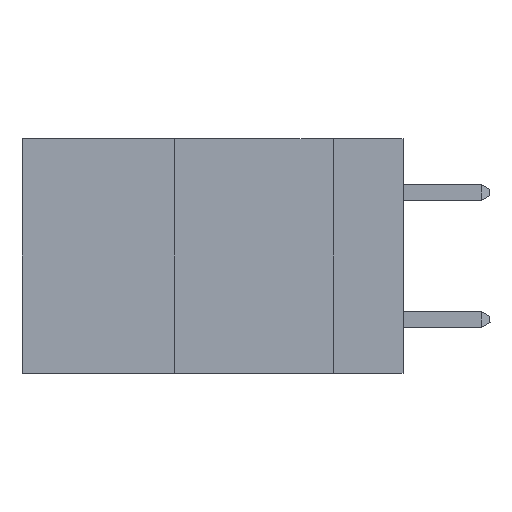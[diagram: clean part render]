
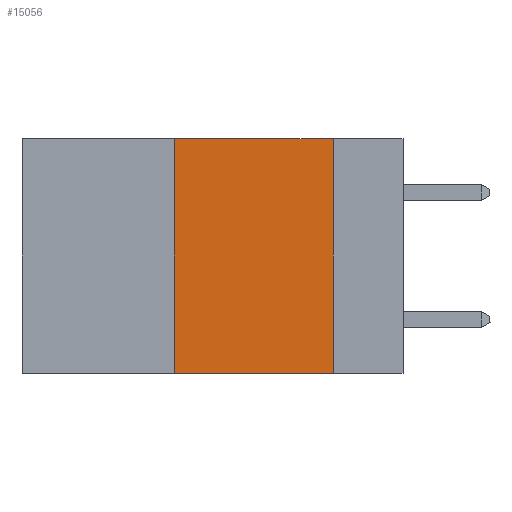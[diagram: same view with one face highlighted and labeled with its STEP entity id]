
A CAD part, left-side view. The second image highlights one B-rep face of the part: STEP entity #15056.
In plain terms, the highlighted planar face has unit normal (-1, 0, 0).
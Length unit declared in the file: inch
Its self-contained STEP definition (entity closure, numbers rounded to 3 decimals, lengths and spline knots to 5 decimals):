
#1637 = LINE ( 'NONE', #20381, #5065 ) ;
#2630 = EDGE_CURVE ( 'NONE', #11672, #5572, #18653, .T. ) ;
#3576 = CARTESIAN_POINT ( 'NONE',  ( 0., 0.36, 0. ) ) ;
#3713 = ORIENTED_EDGE ( 'NONE', *, *, #13079, .F. ) ;
#3814 = ORIENTED_EDGE ( 'NONE', *, *, #17910, .F. ) ;
#4360 = CARTESIAN_POINT ( 'NONE',  ( 0., 0.11, 0. ) ) ;
#4587 = CARTESIAN_POINT ( 'NONE',  ( 0., 0.36, -0.37 ) ) ;
#4958 = LINE ( 'NONE', #16543, #14287 ) ;
#5065 = VECTOR ( 'NONE', #20529, 39.37008 ) ;
#5572 = VERTEX_POINT ( 'NONE', #16097 ) ;
#6463 = CARTESIAN_POINT ( 'NONE',  ( 0., 0.6, -0.37 ) ) ;
#6988 = AXIS2_PLACEMENT_3D ( 'NONE', #13188, #16568, #13337 ) ;
#8141 = VERTEX_POINT ( 'NONE', #4587 ) ;
#8679 = FACE_OUTER_BOUND ( 'NONE', #17442, .T. ) ;
#9706 = DIRECTION ( 'NONE',  ( 0., -1., 0. ) ) ;
#10483 = ORIENTED_EDGE ( 'NONE', *, *, #20546, .T. ) ;
#10667 = ORIENTED_EDGE ( 'NONE', *, *, #2630, .F. ) ;
#11643 = PLANE ( 'NONE',  #6988 ) ;
#11672 = VERTEX_POINT ( 'NONE', #21267 ) ;
#13079 = EDGE_CURVE ( 'NONE', #8141, #15385, #4958, .T. ) ;
#13188 = CARTESIAN_POINT ( 'NONE',  ( 0., 0.6, 0. ) ) ;
#13337 = DIRECTION ( 'NONE',  ( 0., 0., -1. ) ) ;
#14287 = VECTOR ( 'NONE', #19922, 39.37008 ) ;
#15056 = ADVANCED_FACE ( 'NONE', ( #8679 ), #11643, .F. ) ;
#15298 = LINE ( 'NONE', #6463, #15627 ) ;
#15385 = VERTEX_POINT ( 'NONE', #3576 ) ;
#15627 = VECTOR ( 'NONE', #9706, 39.37008 ) ;
#16097 = CARTESIAN_POINT ( 'NONE',  ( 0., 0.11, -0.37 ) ) ;
#16543 = CARTESIAN_POINT ( 'NONE',  ( 0., 0.36, 0. ) ) ;
#16568 = DIRECTION ( 'NONE',  ( 1., 0., 0. ) ) ;
#17442 = EDGE_LOOP ( 'NONE', ( #10667, #3814, #3713, #10483 ) ) ;
#17910 = EDGE_CURVE ( 'NONE', #15385, #11672, #1637, .T. ) ;
#18653 = LINE ( 'NONE', #4360, #21596 ) ;
#19922 = DIRECTION ( 'NONE',  ( 0., 0., 1. ) ) ;
#20381 = CARTESIAN_POINT ( 'NONE',  ( 0., 0.6, 0. ) ) ;
#20529 = DIRECTION ( 'NONE',  ( 0., -1., 0. ) ) ;
#20546 = EDGE_CURVE ( 'NONE', #8141, #5572, #15298, .T. ) ;
#21211 = DIRECTION ( 'NONE',  ( 0., 0., -1. ) ) ;
#21267 = CARTESIAN_POINT ( 'NONE',  ( 0., 0.11, 0. ) ) ;
#21596 = VECTOR ( 'NONE', #21211, 39.37008 ) ;
